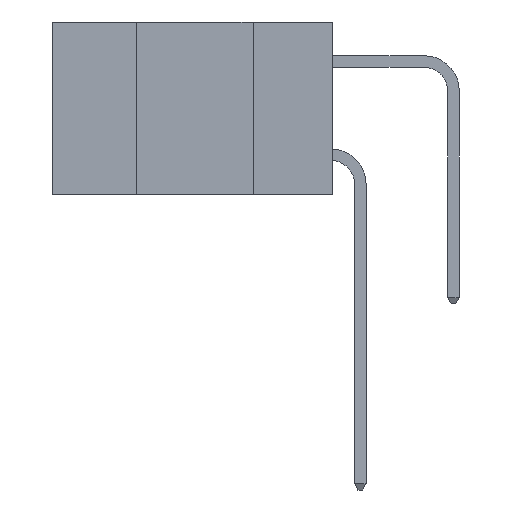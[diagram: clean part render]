
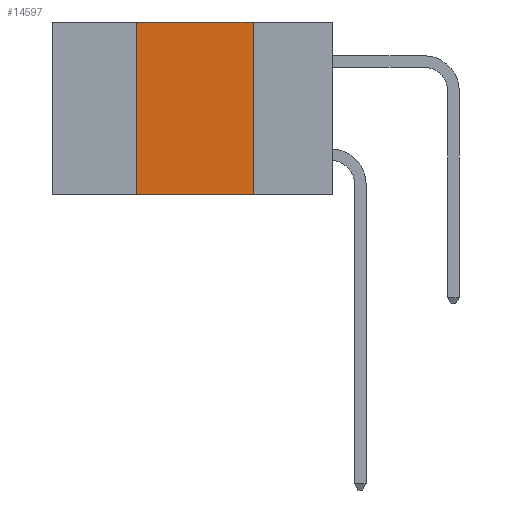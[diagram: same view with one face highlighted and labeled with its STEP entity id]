
A CAD part, left-side view. The second image highlights one B-rep face of the part: STEP entity #14597.
In plain terms, the highlighted planar face has unit normal (-1, 0, 0).
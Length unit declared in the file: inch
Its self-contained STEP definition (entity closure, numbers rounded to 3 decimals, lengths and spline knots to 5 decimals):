
#983 = EDGE_CURVE ( 'NONE', #14802, #11470, #7440, .T. ) ;
#1745 = VERTEX_POINT ( 'NONE', #6850 ) ;
#1952 = EDGE_CURVE ( 'NONE', #11470, #1745, #14031, .T. ) ;
#2154 = AXIS2_PLACEMENT_3D ( 'NONE', #16409, #4632, #13942 ) ;
#2215 = CARTESIAN_POINT ( 'NONE',  ( 0., 0.42, 0. ) ) ;
#2602 = DIRECTION ( 'NONE',  ( 0., 0., -1. ) ) ;
#2782 = CARTESIAN_POINT ( 'NONE',  ( 0., 0.17, -0.37 ) ) ;
#2980 = ORIENTED_EDGE ( 'NONE', *, *, #9514, .F. ) ;
#3330 = CARTESIAN_POINT ( 'NONE',  ( 0., 0.42, -0.37 ) ) ;
#3769 = LINE ( 'NONE', #12173, #7407 ) ;
#4281 = VECTOR ( 'NONE', #7782, 39.37008 ) ;
#4632 = DIRECTION ( 'NONE',  ( 1., 0., 0. ) ) ;
#4860 = VERTEX_POINT ( 'NONE', #3330 ) ;
#5056 = CARTESIAN_POINT ( 'NONE',  ( 0., 0.6, 0. ) ) ;
#5794 = ORIENTED_EDGE ( 'NONE', *, *, #1952, .F. ) ;
#6394 = DIRECTION ( 'NONE',  ( 0., -1., 0. ) ) ;
#6500 = CARTESIAN_POINT ( 'NONE',  ( 0., 0.6, -0.37 ) ) ;
#6850 = CARTESIAN_POINT ( 'NONE',  ( 0., 0.17, -0.37 ) ) ;
#7407 = VECTOR ( 'NONE', #12138, 39.37008 ) ;
#7440 = LINE ( 'NONE', #5056, #16998 ) ;
#7782 = DIRECTION ( 'NONE',  ( 0., -1., 0. ) ) ;
#8252 = LINE ( 'NONE', #6500, #4281 ) ;
#9514 = EDGE_CURVE ( 'NONE', #4860, #14802, #3769, .T. ) ;
#10455 = VECTOR ( 'NONE', #2602, 39.37008 ) ;
#11470 = VERTEX_POINT ( 'NONE', #15517 ) ;
#12138 = DIRECTION ( 'NONE',  ( 0., 0., 1. ) ) ;
#12173 = CARTESIAN_POINT ( 'NONE',  ( 0., 0.42, -0.37 ) ) ;
#12593 = PLANE ( 'NONE',  #2154 ) ;
#12848 = ORIENTED_EDGE ( 'NONE', *, *, #983, .F. ) ;
#13202 = EDGE_LOOP ( 'NONE', ( #5794, #12848, #2980, #14097 ) ) ;
#13942 = DIRECTION ( 'NONE',  ( 0., 0., -1. ) ) ;
#14031 = LINE ( 'NONE', #2782, #10455 ) ;
#14097 = ORIENTED_EDGE ( 'NONE', *, *, #14867, .T. ) ;
#14597 = ADVANCED_FACE ( 'NONE', ( #15855 ), #12593, .F. ) ;
#14802 = VERTEX_POINT ( 'NONE', #2215 ) ;
#14867 = EDGE_CURVE ( 'NONE', #4860, #1745, #8252, .T. ) ;
#15517 = CARTESIAN_POINT ( 'NONE',  ( 0., 0.17, 0. ) ) ;
#15855 = FACE_OUTER_BOUND ( 'NONE', #13202, .T. ) ;
#16409 = CARTESIAN_POINT ( 'NONE',  ( 0., 0.6, 0. ) ) ;
#16998 = VECTOR ( 'NONE', #6394, 39.37008 ) ;
